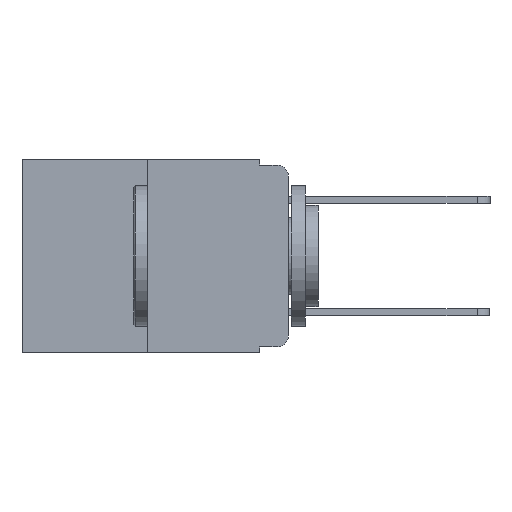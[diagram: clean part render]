
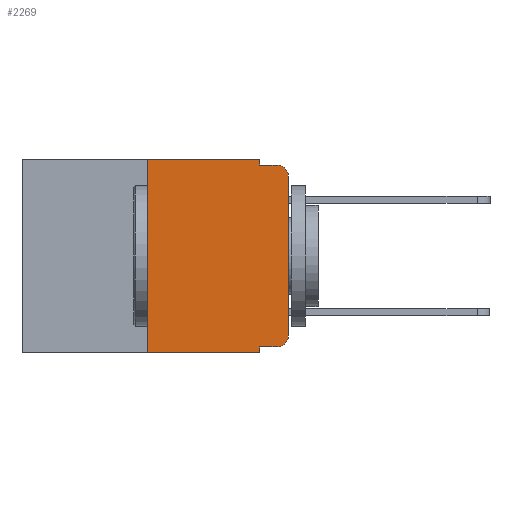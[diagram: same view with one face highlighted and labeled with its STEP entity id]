
A CAD part, left-side view. The second image highlights one B-rep face of the part: STEP entity #2269.
In plain terms, the highlighted planar face has unit normal (-1, 0, 0).
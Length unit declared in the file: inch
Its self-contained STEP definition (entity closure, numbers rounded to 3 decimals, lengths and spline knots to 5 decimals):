
#170 = LINE ( 'NONE', #12006, #9290 ) ;
#352 = VECTOR ( 'NONE', #785, 39.37008 ) ;
#583 = VERTEX_POINT ( 'NONE', #18143 ) ;
#785 = DIRECTION ( 'NONE',  ( 0., 0., -1. ) ) ;
#1060 = CARTESIAN_POINT ( 'NONE',  ( 0., 0.051, 0. ) ) ;
#1720 = EDGE_CURVE ( 'NONE', #17474, #8230, #4422, .T. ) ;
#1896 = EDGE_CURVE ( 'NONE', #583, #12800, #10138, .T. ) ;
#2197 = PLANE ( 'NONE',  #19404 ) ;
#2269 = ADVANCED_FACE ( 'NONE', ( #11273 ), #2197, .F. ) ;
#2286 = DIRECTION ( 'NONE',  ( 0., 0., -1. ) ) ;
#2328 = LINE ( 'NONE', #4286, #16377 ) ;
#2393 = DIRECTION ( 'NONE',  ( 1., 0., 0. ) ) ;
#2672 = CARTESIAN_POINT ( 'NONE',  ( 0., 0.473, 0. ) ) ;
#2790 = ORIENTED_EDGE ( 'NONE', *, *, #3842, .T. ) ;
#2814 = ORIENTED_EDGE ( 'NONE', *, *, #1720, .T. ) ;
#3314 = DIRECTION ( 'NONE',  ( 0., -1., 0. ) ) ;
#3331 = ORIENTED_EDGE ( 'NONE', *, *, #17665, .F. ) ;
#3524 = DIRECTION ( 'NONE',  ( 0., 0., 1. ) ) ;
#3573 = CARTESIAN_POINT ( 'NONE',  ( 0., 0.051, -0.333 ) ) ;
#3592 = DIRECTION ( 'NONE',  ( 0., 0., -1. ) ) ;
#3781 = ORIENTED_EDGE ( 'NONE', *, *, #19606, .F. ) ;
#3842 = EDGE_CURVE ( 'NONE', #12800, #17474, #2328, .T. ) ;
#4286 = CARTESIAN_POINT ( 'NONE',  ( 0., 0., 0. ) ) ;
#4355 = ORIENTED_EDGE ( 'NONE', *, *, #8657, .F. ) ;
#4375 = ORIENTED_EDGE ( 'NONE', *, *, #22688, .F. ) ;
#4422 = CIRCLE ( 'NONE', #8876, 0.02 ) ;
#4710 = CARTESIAN_POINT ( 'NONE',  ( 0., 0.051, -0.343 ) ) ;
#5132 = CARTESIAN_POINT ( 'NONE',  ( 0., 0.473, 0. ) ) ;
#5151 = LINE ( 'NONE', #17260, #352 ) ;
#5487 = ORIENTED_EDGE ( 'NONE', *, *, #14197, .T. ) ;
#6101 = ORIENTED_EDGE ( 'NONE', *, *, #8956, .F. ) ;
#6258 = LINE ( 'NONE', #1060, #11160 ) ;
#6301 = VECTOR ( 'NONE', #8086, 39.37008 ) ;
#6327 = VECTOR ( 'NONE', #16129, 39.37008 ) ;
#6519 = ORIENTED_EDGE ( 'NONE', *, *, #14643, .T. ) ;
#6540 = ORIENTED_EDGE ( 'NONE', *, *, #1896, .T. ) ;
#6601 = LINE ( 'NONE', #5132, #20020 ) ;
#7131 = CARTESIAN_POINT ( 'NONE',  ( 0., 0.051, -0.01 ) ) ;
#7223 = CARTESIAN_POINT ( 'NONE',  ( 0., 0.02, -0.313 ) ) ;
#7498 = LINE ( 'NONE', #8750, #6327 ) ;
#8086 = DIRECTION ( 'NONE',  ( 0., -1., 0. ) ) ;
#8230 = VERTEX_POINT ( 'NONE', #21914 ) ;
#8503 = DIRECTION ( 'NONE',  ( 0., 0., 1. ) ) ;
#8657 = EDGE_CURVE ( 'NONE', #12269, #11446, #6601, .T. ) ;
#8750 = CARTESIAN_POINT ( 'NONE',  ( 0., 0.473, -0.343 ) ) ;
#8876 = AXIS2_PLACEMENT_3D ( 'NONE', #20031, #11397, #12265 ) ;
#8956 = EDGE_CURVE ( 'NONE', #23415, #14040, #5151, .T. ) ;
#9290 = VECTOR ( 'NONE', #8503, 39.37008 ) ;
#9443 = DIRECTION ( 'NONE',  ( -1., 0., 0. ) ) ;
#10138 = CIRCLE ( 'NONE', #19854, 0.02 ) ;
#10771 = VECTOR ( 'NONE', #23332, 39.37008 ) ;
#11126 = VERTEX_POINT ( 'NONE', #22176 ) ;
#11160 = VECTOR ( 'NONE', #15731, 39.37008 ) ;
#11273 = FACE_OUTER_BOUND ( 'NONE', #11298, .T. ) ;
#11298 = EDGE_LOOP ( 'NONE', ( #2790, #2814, #3331, #3781, #4355, #4375, #5487, #6101, #6519, #6540 ) ) ;
#11397 = DIRECTION ( 'NONE',  ( -1., 0., 0. ) ) ;
#11446 = VERTEX_POINT ( 'NONE', #15803 ) ;
#12006 = CARTESIAN_POINT ( 'NONE',  ( 0., 0.25, 0. ) ) ;
#12265 = DIRECTION ( 'NONE',  ( 0., 0., -1. ) ) ;
#12269 = VERTEX_POINT ( 'NONE', #13954 ) ;
#12587 = CARTESIAN_POINT ( 'NONE',  ( 0., 0.051, -0.01 ) ) ;
#12800 = VERTEX_POINT ( 'NONE', #19081 ) ;
#13954 = CARTESIAN_POINT ( 'NONE',  ( 0., 0.25, 0. ) ) ;
#14040 = VERTEX_POINT ( 'NONE', #4710 ) ;
#14197 = EDGE_CURVE ( 'NONE', #11126, #14040, #7498, .T. ) ;
#14643 = EDGE_CURVE ( 'NONE', #23415, #583, #16106, .T. ) ;
#15731 = DIRECTION ( 'NONE',  ( 0., 0., -1. ) ) ;
#15803 = CARTESIAN_POINT ( 'NONE',  ( 0., 0.051, 0. ) ) ;
#16106 = LINE ( 'NONE', #22539, #6301 ) ;
#16129 = DIRECTION ( 'NONE',  ( 0., -1., 0. ) ) ;
#16377 = VECTOR ( 'NONE', #3524, 39.37008 ) ;
#17260 = CARTESIAN_POINT ( 'NONE',  ( 0., 0.051, 0. ) ) ;
#17474 = VERTEX_POINT ( 'NONE', #17582 ) ;
#17582 = CARTESIAN_POINT ( 'NONE',  ( 0., 0., -0.03 ) ) ;
#17665 = EDGE_CURVE ( 'NONE', #17672, #8230, #19880, .T. ) ;
#17672 = VERTEX_POINT ( 'NONE', #7131 ) ;
#18143 = CARTESIAN_POINT ( 'NONE',  ( 0., 0.02, -0.333 ) ) ;
#19081 = CARTESIAN_POINT ( 'NONE',  ( 0., 0., -0.313 ) ) ;
#19404 = AXIS2_PLACEMENT_3D ( 'NONE', #2672, #2393, #2286 ) ;
#19606 = EDGE_CURVE ( 'NONE', #11446, #17672, #6258, .T. ) ;
#19854 = AXIS2_PLACEMENT_3D ( 'NONE', #7223, #9443, #3592 ) ;
#19880 = LINE ( 'NONE', #12587, #10771 ) ;
#20020 = VECTOR ( 'NONE', #3314, 39.37008 ) ;
#20031 = CARTESIAN_POINT ( 'NONE',  ( 0., 0.02, -0.03 ) ) ;
#21914 = CARTESIAN_POINT ( 'NONE',  ( 0., 0.02, -0.01 ) ) ;
#22176 = CARTESIAN_POINT ( 'NONE',  ( 0., 0.25, -0.343 ) ) ;
#22539 = CARTESIAN_POINT ( 'NONE',  ( 0., 0.051, -0.333 ) ) ;
#22688 = EDGE_CURVE ( 'NONE', #11126, #12269, #170, .T. ) ;
#23332 = DIRECTION ( 'NONE',  ( 0., -1., 0. ) ) ;
#23415 = VERTEX_POINT ( 'NONE', #3573 ) ;
